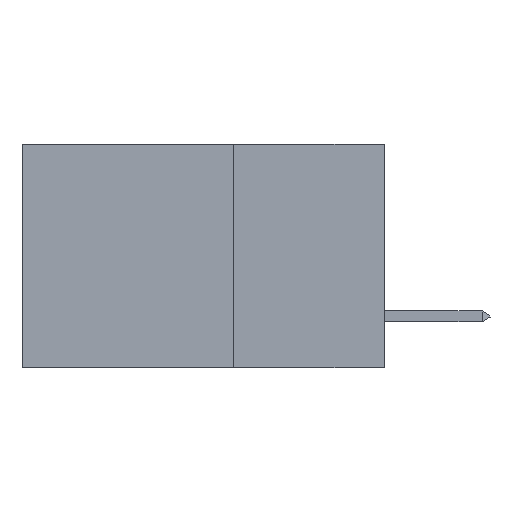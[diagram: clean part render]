
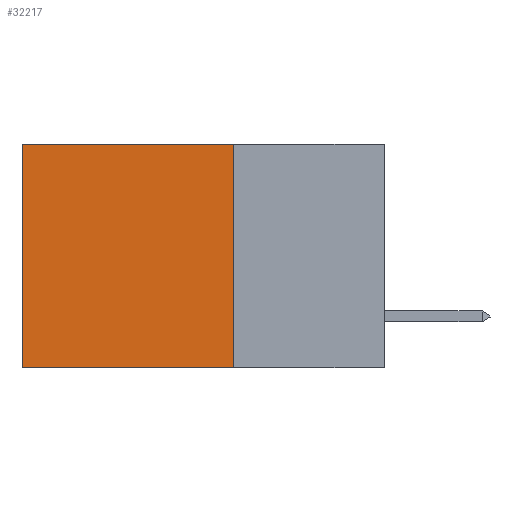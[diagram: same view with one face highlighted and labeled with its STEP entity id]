
A CAD part, left-side view. The second image highlights one B-rep face of the part: STEP entity #32217.
In plain terms, the highlighted planar face has unit normal (-1, 0, 0).
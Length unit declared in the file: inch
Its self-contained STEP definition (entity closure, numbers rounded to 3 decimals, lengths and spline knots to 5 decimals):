
#2922 = VERTEX_POINT ( 'NONE', #9634 ) ;
#2957 = EDGE_CURVE ( 'NONE', #17994, #25125, #19232, .T. ) ;
#4239 = VECTOR ( 'NONE', #15831, 39.37008 ) ;
#4561 = CARTESIAN_POINT ( 'NONE',  ( 0.2875, 0.6, 0. ) ) ;
#7308 = DIRECTION ( 'NONE',  ( 0., 0., -1. ) ) ;
#9634 = CARTESIAN_POINT ( 'NONE',  ( 0.2875, 0.25, 0. ) ) ;
#9692 = EDGE_CURVE ( 'NONE', #29884, #25125, #31931, .T. ) ;
#11340 = VECTOR ( 'NONE', #32853, 39.37008 ) ;
#11656 = LINE ( 'NONE', #12465, #4239 ) ;
#11875 = CARTESIAN_POINT ( 'NONE',  ( 0.2875, 0.25, 0. ) ) ;
#12465 = CARTESIAN_POINT ( 'NONE',  ( 0.2875, 0.25, 0. ) ) ;
#12502 = CARTESIAN_POINT ( 'NONE',  ( 0.2875, 0.6, 0. ) ) ;
#12758 = ORIENTED_EDGE ( 'NONE', *, *, #24356, .F. ) ;
#15516 = EDGE_CURVE ( 'NONE', #2922, #29884, #11656, .T. ) ;
#15831 = DIRECTION ( 'NONE',  ( 0., 1., 0. ) ) ;
#17452 = DIRECTION ( 'NONE',  ( 0., 0., -1. ) ) ;
#17994 = VERTEX_POINT ( 'NONE', #34285 ) ;
#19232 = LINE ( 'NONE', #36902, #11340 ) ;
#20255 = EDGE_LOOP ( 'NONE', ( #36242, #29109, #12758, #28886 ) ) ;
#20692 = FACE_OUTER_BOUND ( 'NONE', #20255, .T. ) ;
#24021 = VECTOR ( 'NONE', #7308, 39.37008 ) ;
#24356 = EDGE_CURVE ( 'NONE', #2922, #17994, #32140, .T. ) ;
#24412 = CARTESIAN_POINT ( 'NONE',  ( 0.2875, 0.6, -0.37 ) ) ;
#24585 = DIRECTION ( 'NONE',  ( 0., 0., -1. ) ) ;
#25125 = VERTEX_POINT ( 'NONE', #24412 ) ;
#28876 = VECTOR ( 'NONE', #24585, 39.37008 ) ;
#28886 = ORIENTED_EDGE ( 'NONE', *, *, #15516, .T. ) ;
#29109 = ORIENTED_EDGE ( 'NONE', *, *, #2957, .F. ) ;
#29645 = DIRECTION ( 'NONE',  ( 1., 0., 0. ) ) ;
#29884 = VERTEX_POINT ( 'NONE', #12502 ) ;
#30142 = CARTESIAN_POINT ( 'NONE',  ( 0.2875, 0.25, 0. ) ) ;
#31517 = AXIS2_PLACEMENT_3D ( 'NONE', #11875, #29645, #17452 ) ;
#31931 = LINE ( 'NONE', #4561, #24021 ) ;
#32140 = LINE ( 'NONE', #30142, #28876 ) ;
#32217 = ADVANCED_FACE ( 'NONE', ( #20692 ), #35265, .F. ) ;
#32853 = DIRECTION ( 'NONE',  ( 0., 1., 0. ) ) ;
#34285 = CARTESIAN_POINT ( 'NONE',  ( 0.2875, 0.25, -0.37 ) ) ;
#35265 = PLANE ( 'NONE',  #31517 ) ;
#36242 = ORIENTED_EDGE ( 'NONE', *, *, #9692, .T. ) ;
#36902 = CARTESIAN_POINT ( 'NONE',  ( 0.2875, 0.25, -0.37 ) ) ;
